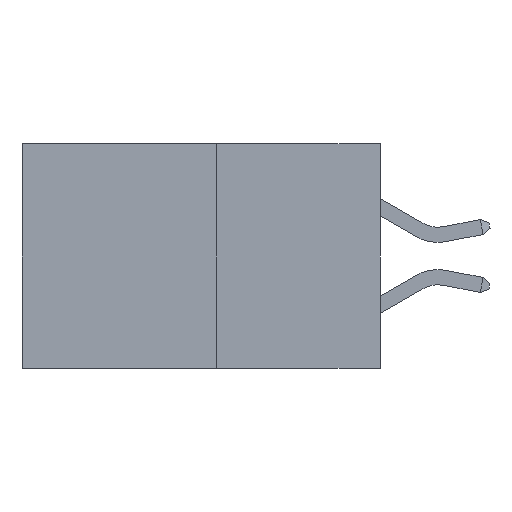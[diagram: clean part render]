
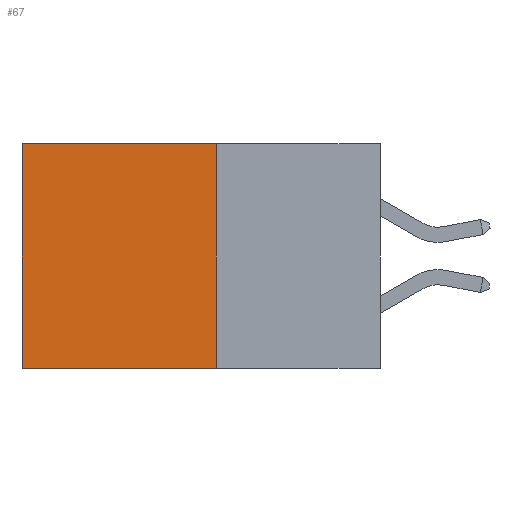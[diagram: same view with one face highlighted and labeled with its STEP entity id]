
A CAD part, left-side view. The second image highlights one B-rep face of the part: STEP entity #67.
In plain terms, the highlighted planar face has unit normal (-1, 0, 0).
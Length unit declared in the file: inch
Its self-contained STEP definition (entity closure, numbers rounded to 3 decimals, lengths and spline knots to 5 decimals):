
#67 = ADVANCED_FACE ( 'NONE', ( #6623 ), #15332, .F. ) ;
#1674 = EDGE_CURVE ( 'NONE', #2153, #3820, #22508, .T. ) ;
#1715 = CARTESIAN_POINT ( 'NONE',  ( 0.277, 0.59, -0.37 ) ) ;
#2153 = VERTEX_POINT ( 'NONE', #12290 ) ;
#2452 = DIRECTION ( 'NONE',  ( 0., 0., -1. ) ) ;
#3820 = VERTEX_POINT ( 'NONE', #1715 ) ;
#4087 = EDGE_CURVE ( 'NONE', #9885, #3820, #13489, .T. ) ;
#6493 = ORIENTED_EDGE ( 'NONE', *, *, #4087, .T. ) ;
#6623 = FACE_OUTER_BOUND ( 'NONE', #19500, .T. ) ;
#6803 = ORIENTED_EDGE ( 'NONE', *, *, #7103, .F. ) ;
#7103 = EDGE_CURVE ( 'NONE', #7189, #2153, #14598, .T. ) ;
#7153 = VECTOR ( 'NONE', #12047, 39.37008 ) ;
#7189 = VERTEX_POINT ( 'NONE', #12793 ) ;
#7388 = LINE ( 'NONE', #19785, #21600 ) ;
#8497 = VECTOR ( 'NONE', #2452, 39.37008 ) ;
#9066 = CARTESIAN_POINT ( 'NONE',  ( 0.277, 0.59, -0.37 ) ) ;
#9885 = VERTEX_POINT ( 'NONE', #16008 ) ;
#9930 = CARTESIAN_POINT ( 'NONE',  ( 0.277, 0.27, -0.37 ) ) ;
#12047 = DIRECTION ( 'NONE',  ( 0., 1., 0. ) ) ;
#12290 = CARTESIAN_POINT ( 'NONE',  ( 0.277, 0.27, -0.37 ) ) ;
#12793 = CARTESIAN_POINT ( 'NONE',  ( 0.277, 0.27, 0. ) ) ;
#13489 = LINE ( 'NONE', #9066, #8497 ) ;
#14275 = DIRECTION ( 'NONE',  ( 0., 0., -1. ) ) ;
#14284 = DIRECTION ( 'NONE',  ( 0., 1., 0. ) ) ;
#14372 = CARTESIAN_POINT ( 'NONE',  ( 0.277, 0.27, -0.37 ) ) ;
#14598 = LINE ( 'NONE', #14372, #23181 ) ;
#15284 = CARTESIAN_POINT ( 'NONE',  ( 0.277, 0.27, -0.37 ) ) ;
#15332 = PLANE ( 'NONE',  #23921 ) ;
#16008 = CARTESIAN_POINT ( 'NONE',  ( 0.277, 0.59, 0. ) ) ;
#16164 = DIRECTION ( 'NONE',  ( 0., 0., -1. ) ) ;
#16224 = DIRECTION ( 'NONE',  ( 1., 0., 0. ) ) ;
#17901 = ORIENTED_EDGE ( 'NONE', *, *, #22659, .T. ) ;
#19500 = EDGE_LOOP ( 'NONE', ( #6493, #23588, #6803, #17901 ) ) ;
#19785 = CARTESIAN_POINT ( 'NONE',  ( 0.277, 0.27, 0. ) ) ;
#21600 = VECTOR ( 'NONE', #14284, 39.37008 ) ;
#22508 = LINE ( 'NONE', #9930, #7153 ) ;
#22659 = EDGE_CURVE ( 'NONE', #7189, #9885, #7388, .T. ) ;
#23181 = VECTOR ( 'NONE', #14275, 39.37008 ) ;
#23588 = ORIENTED_EDGE ( 'NONE', *, *, #1674, .F. ) ;
#23921 = AXIS2_PLACEMENT_3D ( 'NONE', #15284, #16224, #16164 ) ;
